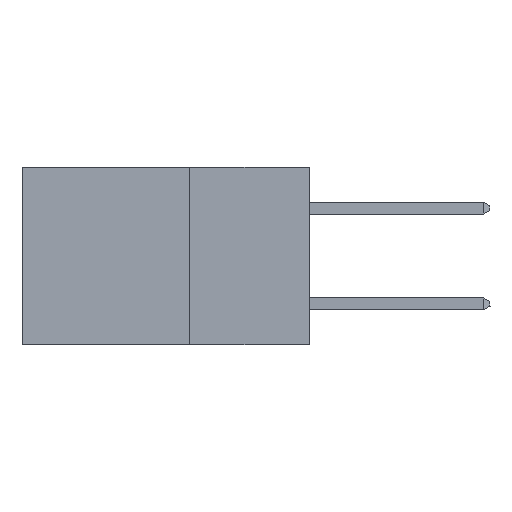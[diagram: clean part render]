
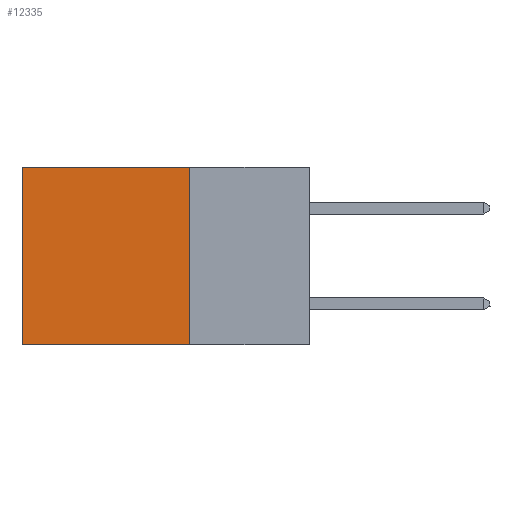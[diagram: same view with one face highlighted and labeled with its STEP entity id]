
A CAD part, left-side view. The second image highlights one B-rep face of the part: STEP entity #12335.
In plain terms, the highlighted planar face has unit normal (-1, 0, 0).
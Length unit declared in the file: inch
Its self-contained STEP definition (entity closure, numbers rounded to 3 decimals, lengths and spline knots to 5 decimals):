
#1138 = CARTESIAN_POINT ( 'NONE',  ( 0.2875, 0.25, 0. ) ) ;
#1321 = VERTEX_POINT ( 'NONE', #13375 ) ;
#1647 = PLANE ( 'NONE',  #5544 ) ;
#1750 = EDGE_CURVE ( 'NONE', #6972, #15222, #17366, .T. ) ;
#1859 = ORIENTED_EDGE ( 'NONE', *, *, #1750, .F. ) ;
#4615 = VECTOR ( 'NONE', #5775, 39.37008 ) ;
#5544 = AXIS2_PLACEMENT_3D ( 'NONE', #14725, #6103, #16135 ) ;
#5603 = DIRECTION ( 'NONE',  ( 0., 1., 0. ) ) ;
#5775 = DIRECTION ( 'NONE',  ( 0., 0., -1. ) ) ;
#6027 = LINE ( 'NONE', #12983, #4615 ) ;
#6103 = DIRECTION ( 'NONE',  ( 1., 0., 0. ) ) ;
#6265 = EDGE_CURVE ( 'NONE', #15543, #1321, #6027, .T. ) ;
#6338 = EDGE_LOOP ( 'NONE', ( #6771, #9755, #1859, #13372 ) ) ;
#6771 = ORIENTED_EDGE ( 'NONE', *, *, #6265, .T. ) ;
#6972 = VERTEX_POINT ( 'NONE', #13076 ) ;
#7790 = VECTOR ( 'NONE', #11596, 39.37008 ) ;
#9341 = FACE_OUTER_BOUND ( 'NONE', #6338, .T. ) ;
#9755 = ORIENTED_EDGE ( 'NONE', *, *, #12220, .F. ) ;
#10969 = CARTESIAN_POINT ( 'NONE',  ( 0.2875, 0.6, 0. ) ) ;
#11596 = DIRECTION ( 'NONE',  ( 0., 1., 0. ) ) ;
#11629 = LINE ( 'NONE', #12994, #7790 ) ;
#12220 = EDGE_CURVE ( 'NONE', #15222, #1321, #11629, .T. ) ;
#12335 = ADVANCED_FACE ( 'NONE', ( #9341 ), #1647, .F. ) ;
#12983 = CARTESIAN_POINT ( 'NONE',  ( 0.2875, 0.6, 0. ) ) ;
#12994 = CARTESIAN_POINT ( 'NONE',  ( 0.2875, 0.25, -0.37 ) ) ;
#13076 = CARTESIAN_POINT ( 'NONE',  ( 0.2875, 0.25, 0. ) ) ;
#13372 = ORIENTED_EDGE ( 'NONE', *, *, #14002, .T. ) ;
#13375 = CARTESIAN_POINT ( 'NONE',  ( 0.2875, 0.6, -0.37 ) ) ;
#13615 = VECTOR ( 'NONE', #18118, 39.37008 ) ;
#14002 = EDGE_CURVE ( 'NONE', #6972, #15543, #17929, .T. ) ;
#14186 = VECTOR ( 'NONE', #5603, 39.37008 ) ;
#14577 = CARTESIAN_POINT ( 'NONE',  ( 0.2875, 0.25, -0.37 ) ) ;
#14725 = CARTESIAN_POINT ( 'NONE',  ( 0.2875, 0.25, 0. ) ) ;
#15222 = VERTEX_POINT ( 'NONE', #14577 ) ;
#15543 = VERTEX_POINT ( 'NONE', #10969 ) ;
#16135 = DIRECTION ( 'NONE',  ( 0., 0., -1. ) ) ;
#17366 = LINE ( 'NONE', #18289, #13615 ) ;
#17929 = LINE ( 'NONE', #1138, #14186 ) ;
#18118 = DIRECTION ( 'NONE',  ( 0., 0., -1. ) ) ;
#18289 = CARTESIAN_POINT ( 'NONE',  ( 0.2875, 0.25, 0. ) ) ;
